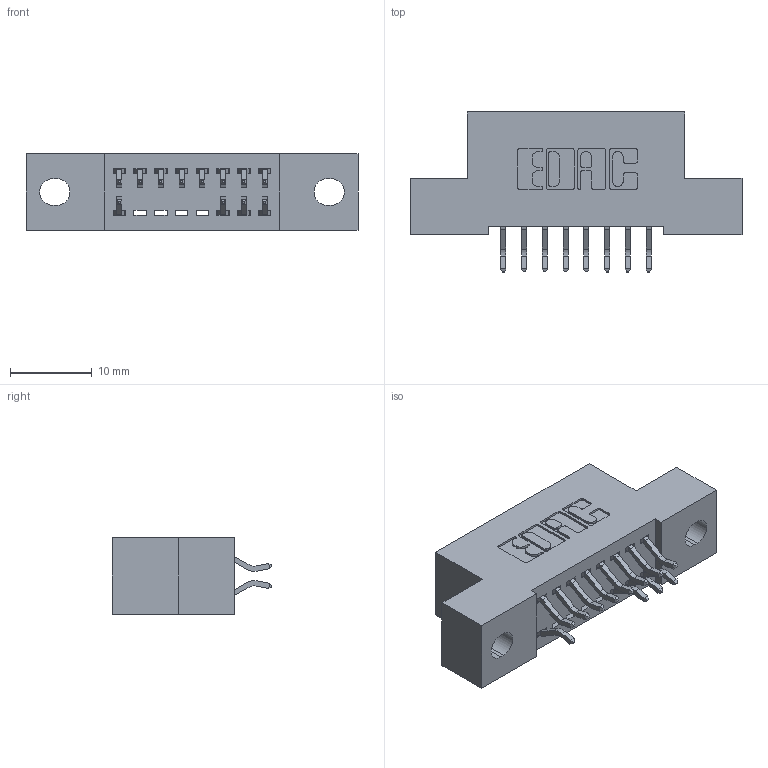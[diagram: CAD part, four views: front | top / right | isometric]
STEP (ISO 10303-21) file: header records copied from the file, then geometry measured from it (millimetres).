
FILE_DESCRIPTION (( 'STEP AP203' ), '1' );
FILE_NAME ('392-016-556-202.STEP', '2018-08-15T02:25:42', ( '' ), ( '' ), 'SwSTEP 2.0', 'SolidWorks 2016', '' );
FILE_SCHEMA (( 'CONFIG_CONTROL_DESIGN' ));
Length unit declared in the file: inch
Products named in the file (3): 345-292-001_556 Tail; 392-016-556-202; 342 Part_.128 Slot
Assembly tree (13 placements, depth 2):
  392-016-556-202
    342 Part_.128 Slot
    345-292-001_556 Tail  x12
Bounding box: 40.64 x 19.58 x 9.4 mm (x, y, z)
Volume: 3402.1 mm3; surface area: 4248.9 mm2
Topology: 13 solids, 13 shells, 834 faces, 2471 edges, 1630 vertices
Faces by surface type: plane 574, cylinder 260
Entity records: 9639 total; most frequent: CARTESIAN_POINT 1670, ORIENTED_EDGE 1598, DIRECTION 1471, EDGE_CURVE 799, LINE 663, VECTOR 663, VERTEX_POINT 530, AXIS2_PLACEMENT_3D 404
